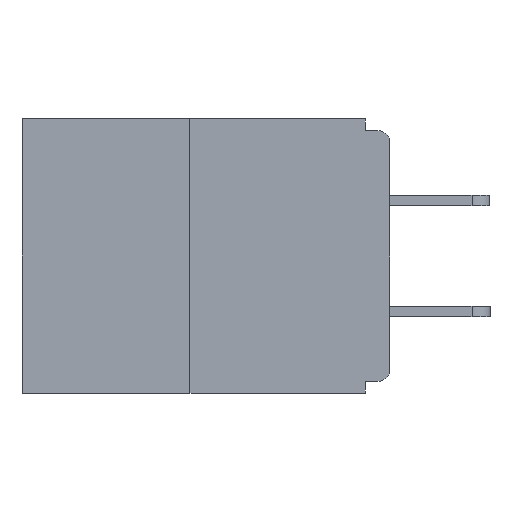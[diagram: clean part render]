
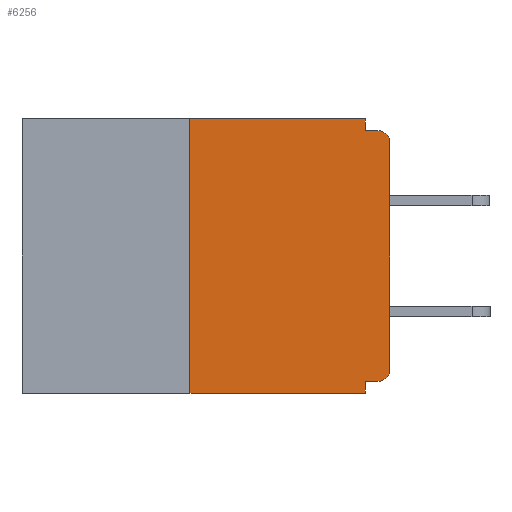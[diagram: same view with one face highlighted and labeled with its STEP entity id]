
A CAD part, left-side view. The second image highlights one B-rep face of the part: STEP entity #6256.
In plain terms, the highlighted planar face has unit normal (-1, 0, 0).
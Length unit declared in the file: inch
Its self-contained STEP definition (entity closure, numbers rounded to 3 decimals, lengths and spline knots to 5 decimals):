
#579 = VECTOR ( 'NONE', #10012, 39.37008 ) ;
#782 = CARTESIAN_POINT ( 'NONE',  ( 0., 0.031, -0.015 ) ) ;
#817 = VECTOR ( 'NONE', #19918, 39.37008 ) ;
#894 = EDGE_CURVE ( 'NONE', #14318, #11749, #13307, .T. ) ;
#1090 = LINE ( 'NONE', #17695, #579 ) ;
#1313 = VERTEX_POINT ( 'NONE', #18183 ) ;
#1429 = ORIENTED_EDGE ( 'NONE', *, *, #8598, .T. ) ;
#1471 = DIRECTION ( 'NONE',  ( 1., 0., 0. ) ) ;
#1598 = LINE ( 'NONE', #18243, #13782 ) ;
#1861 = CIRCLE ( 'NONE', #12643, 0.015 ) ;
#2083 = ORIENTED_EDGE ( 'NONE', *, *, #17298, .F. ) ;
#2480 = DIRECTION ( 'NONE',  ( 0., 0., -1. ) ) ;
#2813 = DIRECTION ( 'NONE',  ( -1., 0., 0. ) ) ;
#3151 = EDGE_CURVE ( 'NONE', #19228, #1313, #16158, .T. ) ;
#3218 = DIRECTION ( 'NONE',  ( 0., 0., -1. ) ) ;
#3597 = CARTESIAN_POINT ( 'NONE',  ( 0., 0.015, -0.328 ) ) ;
#4161 = CARTESIAN_POINT ( 'NONE',  ( 0., 0., -0.015 ) ) ;
#4287 = ORIENTED_EDGE ( 'NONE', *, *, #14970, .F. ) ;
#4463 = AXIS2_PLACEMENT_3D ( 'NONE', #15839, #1471, #19182 ) ;
#4502 = VERTEX_POINT ( 'NONE', #6222 ) ;
#4731 = DIRECTION ( 'NONE',  ( 0., 0., -1. ) ) ;
#5364 = CARTESIAN_POINT ( 'NONE',  ( 0., 0.031, -0.328 ) ) ;
#5371 = VECTOR ( 'NONE', #2480, 39.37008 ) ;
#5735 = VERTEX_POINT ( 'NONE', #19354 ) ;
#5942 = ORIENTED_EDGE ( 'NONE', *, *, #12512, .T. ) ;
#6182 = CARTESIAN_POINT ( 'NONE',  ( 0., 0.25, 0. ) ) ;
#6222 = CARTESIAN_POINT ( 'NONE',  ( 0., 0.015, -0.015 ) ) ;
#6256 = ADVANCED_FACE ( 'NONE', ( #13607 ), #17374, .F. ) ;
#6760 = ORIENTED_EDGE ( 'NONE', *, *, #3151, .F. ) ;
#6875 = LINE ( 'NONE', #8757, #5371 ) ;
#7024 = DIRECTION ( 'NONE',  ( 0., 0., 1. ) ) ;
#7187 = DIRECTION ( 'NONE',  ( 0., -1., 0. ) ) ;
#8207 = DIRECTION ( 'NONE',  ( 0., -1., 0. ) ) ;
#8598 = EDGE_CURVE ( 'NONE', #12530, #5735, #16419, .T. ) ;
#8757 = CARTESIAN_POINT ( 'NONE',  ( 0., 0.031, -0.343 ) ) ;
#8797 = EDGE_LOOP ( 'NONE', ( #6760, #14883, #1429, #2083, #13452, #19002, #5942, #16086, #10048, #4287 ) ) ;
#9550 = CARTESIAN_POINT ( 'NONE',  ( 0., 0.015, -0.313 ) ) ;
#10012 = DIRECTION ( 'NONE',  ( 0., 1., 0. ) ) ;
#10048 = ORIENTED_EDGE ( 'NONE', *, *, #12633, .F. ) ;
#10701 = DIRECTION ( 'NONE',  ( 0., -1., 0. ) ) ;
#10793 = AXIS2_PLACEMENT_3D ( 'NONE', #9550, #11154, #3218 ) ;
#10960 = VECTOR ( 'NONE', #4731, 39.37008 ) ;
#11154 = DIRECTION ( 'NONE',  ( -1., 0., 0. ) ) ;
#11264 = CARTESIAN_POINT ( 'NONE',  ( 0., 0., -0.313 ) ) ;
#11431 = VERTEX_POINT ( 'NONE', #5364 ) ;
#11506 = VECTOR ( 'NONE', #8207, 39.37008 ) ;
#11749 = VERTEX_POINT ( 'NONE', #11264 ) ;
#11812 = LINE ( 'NONE', #16700, #817 ) ;
#11954 = CARTESIAN_POINT ( 'NONE',  ( 0., 0.25, -0.343 ) ) ;
#12269 = EDGE_CURVE ( 'NONE', #14318, #11431, #1090, .T. ) ;
#12491 = EDGE_CURVE ( 'NONE', #12530, #19228, #11812, .T. ) ;
#12512 = EDGE_CURVE ( 'NONE', #11749, #13565, #1598, .T. ) ;
#12530 = VERTEX_POINT ( 'NONE', #11954 ) ;
#12633 = EDGE_CURVE ( 'NONE', #15146, #4502, #19714, .T. ) ;
#12643 = AXIS2_PLACEMENT_3D ( 'NONE', #20244, #2813, #18860 ) ;
#13307 = CIRCLE ( 'NONE', #10793, 0.015 ) ;
#13452 = ORIENTED_EDGE ( 'NONE', *, *, #12269, .F. ) ;
#13565 = VERTEX_POINT ( 'NONE', #16398 ) ;
#13607 = FACE_OUTER_BOUND ( 'NONE', #8797, .T. ) ;
#13642 = CARTESIAN_POINT ( 'NONE',  ( 0., 0.46, 0. ) ) ;
#13782 = VECTOR ( 'NONE', #7024, 39.37008 ) ;
#14318 = VERTEX_POINT ( 'NONE', #3597 ) ;
#14883 = ORIENTED_EDGE ( 'NONE', *, *, #12491, .F. ) ;
#14970 = EDGE_CURVE ( 'NONE', #1313, #15146, #18628, .T. ) ;
#15146 = VERTEX_POINT ( 'NONE', #782 ) ;
#15804 = CARTESIAN_POINT ( 'NONE',  ( 0., 0.031, 0. ) ) ;
#15839 = CARTESIAN_POINT ( 'NONE',  ( 0., 0.46, 0. ) ) ;
#16086 = ORIENTED_EDGE ( 'NONE', *, *, #18185, .T. ) ;
#16158 = LINE ( 'NONE', #13642, #17637 ) ;
#16398 = CARTESIAN_POINT ( 'NONE',  ( 0., 0., -0.03 ) ) ;
#16419 = LINE ( 'NONE', #17622, #11506 ) ;
#16700 = CARTESIAN_POINT ( 'NONE',  ( 0., 0.25, 0. ) ) ;
#17298 = EDGE_CURVE ( 'NONE', #11431, #5735, #6875, .T. ) ;
#17374 = PLANE ( 'NONE',  #4463 ) ;
#17622 = CARTESIAN_POINT ( 'NONE',  ( 0., 0.46, -0.343 ) ) ;
#17637 = VECTOR ( 'NONE', #7187, 39.37008 ) ;
#17695 = CARTESIAN_POINT ( 'NONE',  ( 0., 0., -0.328 ) ) ;
#18183 = CARTESIAN_POINT ( 'NONE',  ( 0., 0.031, 0. ) ) ;
#18185 = EDGE_CURVE ( 'NONE', #13565, #4502, #1861, .T. ) ;
#18243 = CARTESIAN_POINT ( 'NONE',  ( 0., 0., 0. ) ) ;
#18628 = LINE ( 'NONE', #15804, #10960 ) ;
#18860 = DIRECTION ( 'NONE',  ( 0., 0., -1. ) ) ;
#18959 = VECTOR ( 'NONE', #10701, 39.37008 ) ;
#19002 = ORIENTED_EDGE ( 'NONE', *, *, #894, .T. ) ;
#19182 = DIRECTION ( 'NONE',  ( 0., 0., -1. ) ) ;
#19228 = VERTEX_POINT ( 'NONE', #6182 ) ;
#19354 = CARTESIAN_POINT ( 'NONE',  ( 0., 0.031, -0.343 ) ) ;
#19714 = LINE ( 'NONE', #4161, #18959 ) ;
#19918 = DIRECTION ( 'NONE',  ( 0., 0., 1. ) ) ;
#20244 = CARTESIAN_POINT ( 'NONE',  ( 0., 0.015, -0.03 ) ) ;
